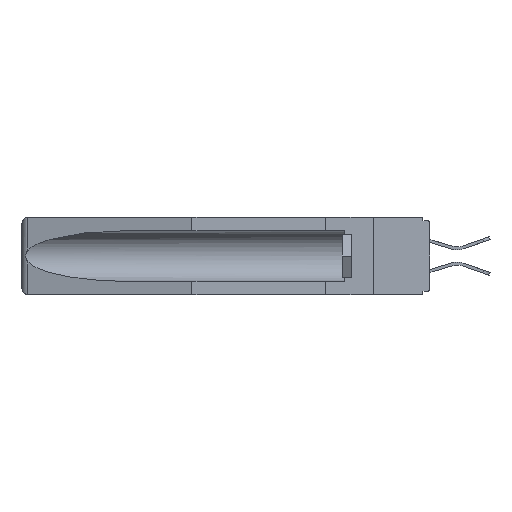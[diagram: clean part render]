
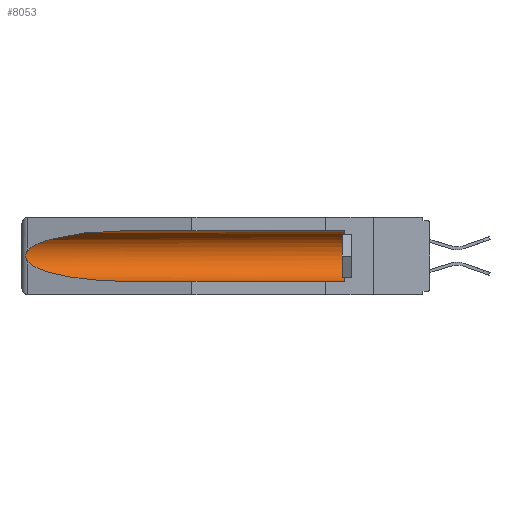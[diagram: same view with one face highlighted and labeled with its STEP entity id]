
A CAD part, left-side view. The second image highlights one B-rep face of the part: STEP entity #8053.
In plain terms, the highlighted cylindrical face has radius 2.857 mm (diameter 5.715 mm), a partial arc.
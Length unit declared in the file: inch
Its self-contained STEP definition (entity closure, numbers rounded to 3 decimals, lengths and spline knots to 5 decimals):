
#568 = CARTESIAN_POINT ( 'NONE',  ( 0.21114, 1.30732, -0.284 ) ) ;
#596 = LINE ( 'NONE', #2296, #16910 ) ;
#1256 = DIRECTION ( 'NONE',  ( 0., -1., 0. ) ) ;
#1524 = CARTESIAN_POINT ( 'NONE',  ( 0.26597, 1.5296, -0.19026 ) ) ;
#1699 = CARTESIAN_POINT ( 'NONE',  ( 0.155, 1.07973, -0.059 ) ) ;
#2296 = CARTESIAN_POINT ( 'NONE',  ( 0.155, -0.30754, -0.059 ) ) ;
#3170 = EDGE_CURVE ( 'NONE', #5956, #10614, #18939, .T. ) ;
#4163 = CARTESIAN_POINT ( 'NONE',  ( 0.26597, 1.52961, -0.15275 ) ) ;
#4280 = CARTESIAN_POINT ( 'NONE',  ( 0.2673, 1.53269, -0.17917 ) ) ;
#4738 = CARTESIAN_POINT ( 'NONE',  ( 0.25451, 1.48313, -0.09465 ) ) ;
#5073 = VECTOR ( 'NONE', #28778, 39.37008 ) ;
#5923 = EDGE_LOOP ( 'NONE', ( #27683, #24588, #23192, #31362, #23775, #26951 ) ) ;
#5956 = VERTEX_POINT ( 'NONE', #11845 ) ;
#6537 = CARTESIAN_POINT ( 'NONE',  ( 0.26537, 1.52718, -0.19328 ) ) ;
#6641 = CARTESIAN_POINT ( 'NONE',  ( 0.2675, 1.53308, -0.16763 ) ) ;
#7913 = EDGE_CURVE ( 'NONE', #12678, #32035, #18257, .T. ) ;
#8053 = ADVANCED_FACE ( 'NONE', ( #28309 ), #14752, .F. ) ;
#8238 = CARTESIAN_POINT ( 'NONE',  ( 0.155, 0.126, -0.284 ) ) ;
#8505 = CARTESIAN_POINT ( 'NONE',  ( 0.25451, 1.48313, -0.24835 ) ) ;
#9612 = EDGE_CURVE ( 'NONE', #11613, #10760, #596, .T. ) ;
#9620 = AXIS2_PLACEMENT_3D ( 'NONE', #31041, #1256, #18652 ) ;
#10614 = VERTEX_POINT ( 'NONE', #26559 ) ;
#10760 = VERTEX_POINT ( 'NONE', #1699 ) ;
#11613 = VERTEX_POINT ( 'NONE', #26966 ) ;
#11634 = CARTESIAN_POINT ( 'NONE',  ( 0.26654, 1.53092, -0.15636 ) ) ;
#11845 = CARTESIAN_POINT ( 'NONE',  ( 0.26537, 1.52718, -0.14972 ) ) ;
#11941 = CARTESIAN_POINT ( 'NONE',  ( 0.155, -0.30754, -0.1715 ) ) ;
#11976 = CIRCLE ( 'NONE', #9620, 0.1125 ) ;
#12678 = VERTEX_POINT ( 'NONE', #8238 ) ;
#12980 = CARTESIAN_POINT ( 'NONE',  ( 0.155, 1.07973, -0.284 ) ) ;
#14194 = CARTESIAN_POINT ( 'NONE',  ( 0.155, -0.30754, -0.284 ) ) ;
#14718 = CARTESIAN_POINT ( 'NONE',  ( 0.155, 1.07973, -0.284 ) ) ;
#14752 = CYLINDRICAL_SURFACE ( 'NONE', #23318, 0.1125 ) ;
#16910 = VECTOR ( 'NONE', #32159, 39.37008 ) ;
#17360 =( BOUNDED_CURVE ( )  B_SPLINE_CURVE ( 3, ( #31876, #21990, #4738, #24164 ),
 .UNSPECIFIED., .F., .F. ) 
 B_SPLINE_CURVE_WITH_KNOTS ( ( 4, 4 ),
 ( 4.71239, 6.08839 ),
 .UNSPECIFIED. ) 
 CURVE ( )  GEOMETRIC_REPRESENTATION_ITEM ( )  RATIONAL_B_SPLINE_CURVE ( ( 1., 0.848, 0.848, 1. ) ) 
 REPRESENTATION_ITEM ( '' )  );
#17446 = DIRECTION ( 'NONE',  ( 0., 0., 1. ) ) ;
#18257 = LINE ( 'NONE', #14194, #5073 ) ;
#18652 = DIRECTION ( 'NONE',  ( 0., 0., 1. ) ) ;
#18939 = B_SPLINE_CURVE_WITH_KNOTS ( 'NONE', 3,
 ( #31292, #4163, #11634, #31412, #6641, #29022, #4280, #21520, #1524, #6537 ),
 .UNSPECIFIED., .F., .F.,
 ( 4, 2, 2, 2, 4 ),
 ( 0., 0.00029, 0.00058, 0.00087, 0.00117 ),
 .UNSPECIFIED. ) ;
#20471 = CARTESIAN_POINT ( 'NONE',  ( 0.26537, 1.52718, -0.19328 ) ) ;
#21520 = CARTESIAN_POINT ( 'NONE',  ( 0.26655, 1.53094, -0.18657 ) ) ;
#21990 = CARTESIAN_POINT ( 'NONE',  ( 0.21114, 1.30732, -0.059 ) ) ;
#23192 = ORIENTED_EDGE ( 'NONE', *, *, #31274, .T. ) ;
#23318 = AXIS2_PLACEMENT_3D ( 'NONE', #11941, #31816, #17446 ) ;
#23775 = ORIENTED_EDGE ( 'NONE', *, *, #23918, .T. ) ;
#23918 = EDGE_CURVE ( 'NONE', #12678, #11613, #11976, .T. ) ;
#24164 = CARTESIAN_POINT ( 'NONE',  ( 0.26537, 1.52718, -0.14972 ) ) ;
#24588 = ORIENTED_EDGE ( 'NONE', *, *, #3170, .T. ) ;
#26559 = CARTESIAN_POINT ( 'NONE',  ( 0.26537, 1.52718, -0.19328 ) ) ;
#26951 = ORIENTED_EDGE ( 'NONE', *, *, #9612, .T. ) ;
#26966 = CARTESIAN_POINT ( 'NONE',  ( 0.155, 0.126, -0.059 ) ) ;
#27546 =( BOUNDED_CURVE ( )  B_SPLINE_CURVE ( 3, ( #20471, #8505, #568, #12980 ),
 .UNSPECIFIED., .F., .F. ) 
 B_SPLINE_CURVE_WITH_KNOTS ( ( 4, 4 ),
 ( 0.1948, 1.5708 ),
 .UNSPECIFIED. ) 
 CURVE ( )  GEOMETRIC_REPRESENTATION_ITEM ( )  RATIONAL_B_SPLINE_CURVE ( ( 1., 0.848, 0.848, 1. ) ) 
 REPRESENTATION_ITEM ( '' )  );
#27683 = ORIENTED_EDGE ( 'NONE', *, *, #28541, .T. ) ;
#28309 = FACE_OUTER_BOUND ( 'NONE', #5923, .T. ) ;
#28541 = EDGE_CURVE ( 'NONE', #10760, #5956, #17360, .T. ) ;
#28778 = DIRECTION ( 'NONE',  ( 0., 1., 0. ) ) ;
#29022 = CARTESIAN_POINT ( 'NONE',  ( 0.2675, 1.53308, -0.17534 ) ) ;
#31041 = CARTESIAN_POINT ( 'NONE',  ( 0.155, 0.126, -0.1715 ) ) ;
#31274 = EDGE_CURVE ( 'NONE', #10614, #32035, #27546, .T. ) ;
#31292 = CARTESIAN_POINT ( 'NONE',  ( 0.26537, 1.52718, -0.14972 ) ) ;
#31362 = ORIENTED_EDGE ( 'NONE', *, *, #7913, .F. ) ;
#31412 = CARTESIAN_POINT ( 'NONE',  ( 0.2673, 1.5327, -0.16383 ) ) ;
#31816 = DIRECTION ( 'NONE',  ( 0., 1., 0. ) ) ;
#31876 = CARTESIAN_POINT ( 'NONE',  ( 0.155, 1.07973, -0.059 ) ) ;
#32035 = VERTEX_POINT ( 'NONE', #14718 ) ;
#32159 = DIRECTION ( 'NONE',  ( 0., 1., 0. ) ) ;
